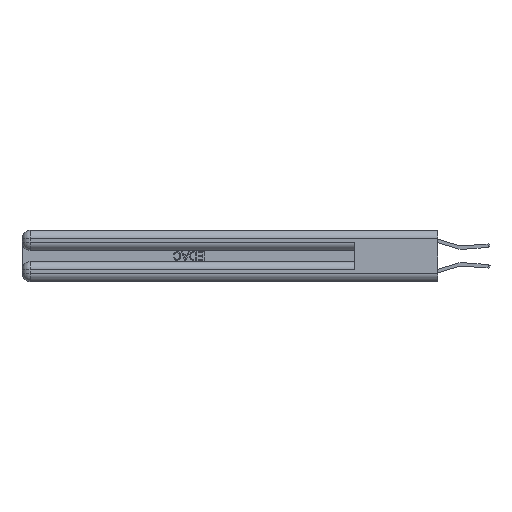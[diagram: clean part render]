
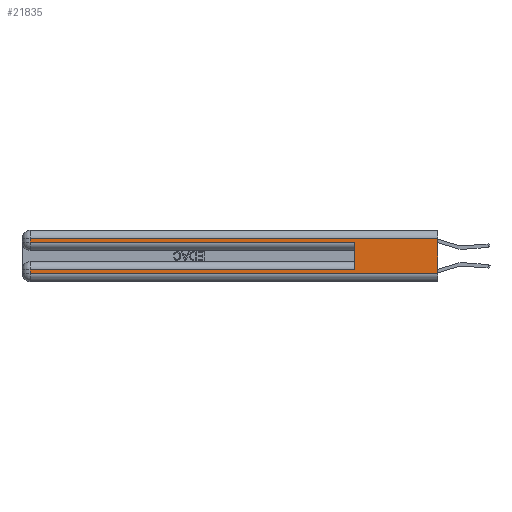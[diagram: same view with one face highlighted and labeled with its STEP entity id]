
A CAD part, left-side view. The second image highlights one B-rep face of the part: STEP entity #21835.
In plain terms, the highlighted planar face has unit normal (-1, 0, 0).
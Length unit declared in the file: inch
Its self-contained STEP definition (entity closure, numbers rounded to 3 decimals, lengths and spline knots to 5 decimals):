
#60 = EDGE_CURVE ( 'NONE', #24457, #31437, #21647, .T. ) ;
#571 = EDGE_CURVE ( 'NONE', #6101, #10160, #13464, .T. ) ;
#758 = CARTESIAN_POINT ( 'NONE',  ( 0., 0., 0.06 ) ) ;
#1279 = LINE ( 'NONE', #35805, #3628 ) ;
#1357 = ORIENTED_EDGE ( 'NONE', *, *, #8248, .T. ) ;
#1732 = DIRECTION ( 'NONE',  ( 0., 0., 1. ) ) ;
#2164 = VECTOR ( 'NONE', #21602, 39.37008 ) ;
#2908 = VECTOR ( 'NONE', #6991, 39.37008 ) ;
#3628 = VECTOR ( 'NONE', #15978, 39.37008 ) ;
#3714 = LINE ( 'NONE', #34854, #15513 ) ;
#3902 = ORIENTED_EDGE ( 'NONE', *, *, #60, .T. ) ;
#5540 = CARTESIAN_POINT ( 'NONE',  ( 0., 2.94, 0.37 ) ) ;
#5963 = ORIENTED_EDGE ( 'NONE', *, *, #32351, .T. ) ;
#6101 = VERTEX_POINT ( 'NONE', #26990 ) ;
#6957 = EDGE_CURVE ( 'NONE', #6101, #11373, #1279, .T. ) ;
#6991 = DIRECTION ( 'NONE',  ( 0., 1., 0. ) ) ;
#7203 = VECTOR ( 'NONE', #28384, 39.37008 ) ;
#7261 = CARTESIAN_POINT ( 'NONE',  ( 0., 2.94, 0.085 ) ) ;
#7290 = CARTESIAN_POINT ( 'NONE',  ( 0., 2.94, 0.37 ) ) ;
#7800 = EDGE_LOOP ( 'NONE', ( #23148, #26051, #5963, #1357, #24741, #18237, #3902, #10585 ) ) ;
#8248 = EDGE_CURVE ( 'NONE', #25712, #24167, #36581, .T. ) ;
#8811 = CARTESIAN_POINT ( 'NONE',  ( 0., 2.94, 0.06 ) ) ;
#10160 = VERTEX_POINT ( 'NONE', #758 ) ;
#10504 = DIRECTION ( 'NONE',  ( 1., 0., 0. ) ) ;
#10585 = ORIENTED_EDGE ( 'NONE', *, *, #16675, .T. ) ;
#11282 = EDGE_CURVE ( 'NONE', #33251, #24457, #32485, .T. ) ;
#11373 = VERTEX_POINT ( 'NONE', #21722 ) ;
#11434 = VECTOR ( 'NONE', #34302, 39.37008 ) ;
#13464 = LINE ( 'NONE', #15723, #2164 ) ;
#13598 = CARTESIAN_POINT ( 'NONE',  ( 0., 0.6, 0.145 ) ) ;
#14245 = CARTESIAN_POINT ( 'NONE',  ( 0., 0., 0.37 ) ) ;
#15513 = VECTOR ( 'NONE', #35215, 39.37008 ) ;
#15723 = CARTESIAN_POINT ( 'NONE',  ( 0., 0., 0.37 ) ) ;
#15802 = EDGE_CURVE ( 'NONE', #33251, #24167, #36654, .T. ) ;
#15978 = DIRECTION ( 'NONE',  ( 0., 1., 0. ) ) ;
#16532 = DIRECTION ( 'NONE',  ( 0., 0., -1. ) ) ;
#16675 = EDGE_CURVE ( 'NONE', #31437, #10160, #3714, .T. ) ;
#16873 = LINE ( 'NONE', #5540, #7203 ) ;
#16926 = CARTESIAN_POINT ( 'NONE',  ( 0., 0.6, 0.085 ) ) ;
#18041 = CARTESIAN_POINT ( 'NONE',  ( 0., 2.94, 0.285 ) ) ;
#18106 = VECTOR ( 'NONE', #1732, 39.37008 ) ;
#18237 = ORIENTED_EDGE ( 'NONE', *, *, #11282, .T. ) ;
#21602 = DIRECTION ( 'NONE',  ( 0., 0., -1. ) ) ;
#21647 = LINE ( 'NONE', #7290, #33505 ) ;
#21722 = CARTESIAN_POINT ( 'NONE',  ( 0., 2.94, 0.31 ) ) ;
#21835 = ADVANCED_FACE ( 'NONE', ( #28607 ), #34102, .F. ) ;
#22235 = CARTESIAN_POINT ( 'NONE',  ( 0., 0., 0.285 ) ) ;
#23148 = ORIENTED_EDGE ( 'NONE', *, *, #571, .F. ) ;
#24167 = VERTEX_POINT ( 'NONE', #33187 ) ;
#24457 = VERTEX_POINT ( 'NONE', #7261 ) ;
#24741 = ORIENTED_EDGE ( 'NONE', *, *, #15802, .F. ) ;
#25712 = VERTEX_POINT ( 'NONE', #18041 ) ;
#26051 = ORIENTED_EDGE ( 'NONE', *, *, #6957, .T. ) ;
#26990 = CARTESIAN_POINT ( 'NONE',  ( 0., 0., 0.31 ) ) ;
#28384 = DIRECTION ( 'NONE',  ( 0., 0., -1. ) ) ;
#28607 = FACE_OUTER_BOUND ( 'NONE', #7800, .T. ) ;
#29159 = DIRECTION ( 'NONE',  ( 0., 0., -1. ) ) ;
#31437 = VERTEX_POINT ( 'NONE', #8811 ) ;
#32351 = EDGE_CURVE ( 'NONE', #11373, #25712, #16873, .T. ) ;
#32485 = LINE ( 'NONE', #35094, #2908 ) ;
#33187 = CARTESIAN_POINT ( 'NONE',  ( 0., 0.6, 0.285 ) ) ;
#33251 = VERTEX_POINT ( 'NONE', #16926 ) ;
#33505 = VECTOR ( 'NONE', #16532, 39.37008 ) ;
#34102 = PLANE ( 'NONE',  #35915 ) ;
#34302 = DIRECTION ( 'NONE',  ( 0., -1., 0. ) ) ;
#34854 = CARTESIAN_POINT ( 'NONE',  ( 0., 0., 0.06 ) ) ;
#35094 = CARTESIAN_POINT ( 'NONE',  ( 0., 0., 0.085 ) ) ;
#35215 = DIRECTION ( 'NONE',  ( 0., -1., 0. ) ) ;
#35805 = CARTESIAN_POINT ( 'NONE',  ( 0., 0., 0.31 ) ) ;
#35915 = AXIS2_PLACEMENT_3D ( 'NONE', #14245, #10504, #29159 ) ;
#36581 = LINE ( 'NONE', #22235, #11434 ) ;
#36654 = LINE ( 'NONE', #13598, #18106 ) ;
